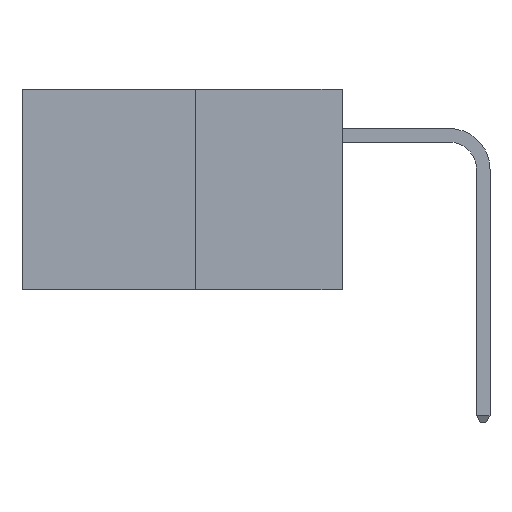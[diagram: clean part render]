
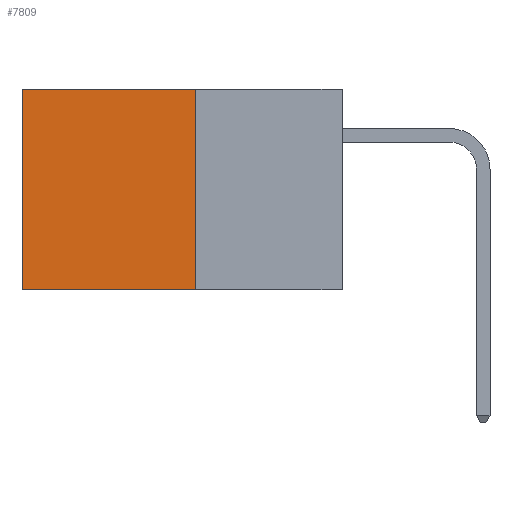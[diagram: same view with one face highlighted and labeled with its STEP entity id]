
A CAD part, left-side view. The second image highlights one B-rep face of the part: STEP entity #7809.
In plain terms, the highlighted planar face has unit normal (-1, 0, 0).
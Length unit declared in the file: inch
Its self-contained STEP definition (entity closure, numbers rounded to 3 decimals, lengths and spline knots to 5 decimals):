
#410 = LINE ( 'NONE', #7906, #5414 ) ;
#677 = EDGE_CURVE ( 'NONE', #1365, #2537, #4643, .T. ) ;
#723 = ORIENTED_EDGE ( 'NONE', *, *, #7526, .F. ) ;
#866 = CARTESIAN_POINT ( 'NONE',  ( 0.277, 0.27, -0.37 ) ) ;
#932 = ORIENTED_EDGE ( 'NONE', *, *, #3634, .F. ) ;
#1121 = VECTOR ( 'NONE', #5834, 39.37008 ) ;
#1284 = DIRECTION ( 'NONE',  ( 0., 0., -1. ) ) ;
#1293 = DIRECTION ( 'NONE',  ( 1., 0., 0. ) ) ;
#1304 = CARTESIAN_POINT ( 'NONE',  ( 0.277, 0.27, -0.37 ) ) ;
#1351 = PLANE ( 'NONE',  #7257 ) ;
#1365 = VERTEX_POINT ( 'NONE', #4649 ) ;
#1398 = ORIENTED_EDGE ( 'NONE', *, *, #3332, .T. ) ;
#1530 = CARTESIAN_POINT ( 'NONE',  ( 0.277, 0.59, -0.37 ) ) ;
#1569 = DIRECTION ( 'NONE',  ( 0., 0., -1. ) ) ;
#2511 = DIRECTION ( 'NONE',  ( 0., 1., 0. ) ) ;
#2537 = VERTEX_POINT ( 'NONE', #1530 ) ;
#2546 = ORIENTED_EDGE ( 'NONE', *, *, #677, .T. ) ;
#2548 = CARTESIAN_POINT ( 'NONE',  ( 0.277, 0.27, -0.37 ) ) ;
#2747 = VECTOR ( 'NONE', #1569, 39.37008 ) ;
#3012 = LINE ( 'NONE', #6583, #1121 ) ;
#3310 = LINE ( 'NONE', #2548, #8268 ) ;
#3332 = EDGE_CURVE ( 'NONE', #6876, #1365, #410, .T. ) ;
#3634 = EDGE_CURVE ( 'NONE', #6876, #5364, #3012, .T. ) ;
#4427 = FACE_OUTER_BOUND ( 'NONE', #5177, .T. ) ;
#4540 = CARTESIAN_POINT ( 'NONE',  ( 0.277, 0.59, -0.37 ) ) ;
#4643 = LINE ( 'NONE', #4540, #2747 ) ;
#4649 = CARTESIAN_POINT ( 'NONE',  ( 0.277, 0.59, 0. ) ) ;
#5177 = EDGE_LOOP ( 'NONE', ( #2546, #723, #932, #1398 ) ) ;
#5364 = VERTEX_POINT ( 'NONE', #866 ) ;
#5414 = VECTOR ( 'NONE', #7890, 39.37008 ) ;
#5730 = CARTESIAN_POINT ( 'NONE',  ( 0.277, 0.27, 0. ) ) ;
#5834 = DIRECTION ( 'NONE',  ( 0., 0., -1. ) ) ;
#6583 = CARTESIAN_POINT ( 'NONE',  ( 0.277, 0.27, -0.37 ) ) ;
#6876 = VERTEX_POINT ( 'NONE', #5730 ) ;
#7257 = AXIS2_PLACEMENT_3D ( 'NONE', #1304, #1293, #1284 ) ;
#7526 = EDGE_CURVE ( 'NONE', #5364, #2537, #3310, .T. ) ;
#7809 = ADVANCED_FACE ( 'NONE', ( #4427 ), #1351, .F. ) ;
#7890 = DIRECTION ( 'NONE',  ( 0., 1., 0. ) ) ;
#7906 = CARTESIAN_POINT ( 'NONE',  ( 0.277, 0.27, 0. ) ) ;
#8268 = VECTOR ( 'NONE', #2511, 39.37008 ) ;
